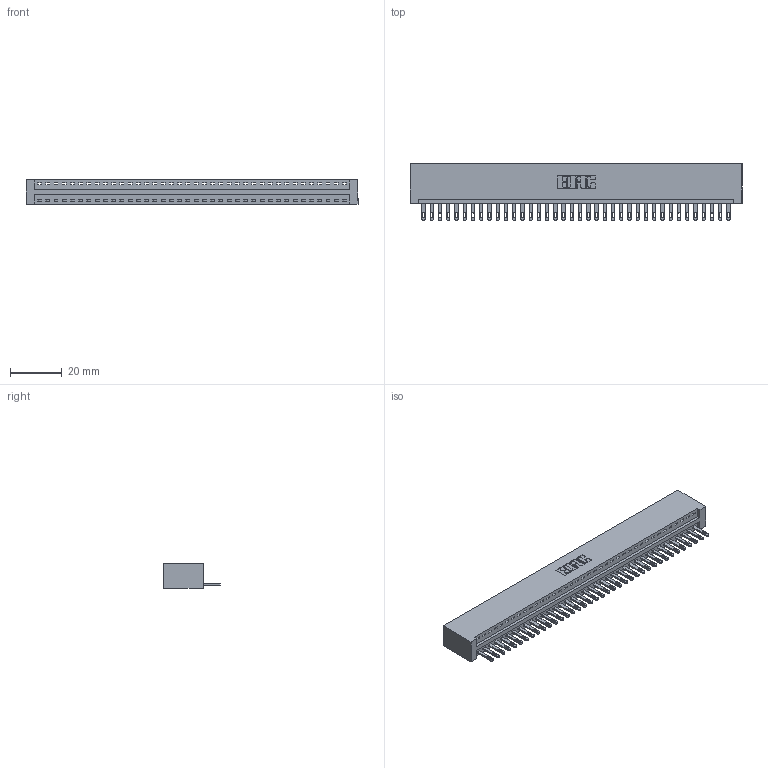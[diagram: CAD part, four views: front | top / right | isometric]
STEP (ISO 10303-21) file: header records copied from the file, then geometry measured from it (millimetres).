
FILE_DESCRIPTION (( 'STEP AP203' ), '1' );
FILE_NAME ('346-038-500-101.STEP', '2022-05-07T03:54:42', ( '' ), ( '' ), 'SwSTEP 2.0', 'SolidWorks 2020', '' );
FILE_SCHEMA (( 'CONFIG_CONTROL_DESIGN' ));
Length unit declared in the file: inch
Products named in the file (3): 346-038-500-101; 346 Part_No Mounting Lugs; 345-292-001_345-293-100
Assembly tree (39 placements, depth 2):
  346-038-500-101
    346 Part_No Mounting Lugs
    345-292-001_345-293-100  x38
Bounding box: 127.89 x 21.84 x 9.4 mm (x, y, z)
Volume: 12787.2 mm3; surface area: 16102.8 mm2
Topology: 39 solids, 39 shells, 2166 faces, 6689 edges, 4458 vertices
Faces by surface type: plane 1364, cylinder 802
Entity records: 23775 total; most frequent: CARTESIAN_POINT 4082, ORIENTED_EDGE 4054, DIRECTION 3603, EDGE_CURVE 2027, VECTOR 1747, LINE 1747, VERTEX_POINT 1350, AXIS2_PLACEMENT_3D 928
